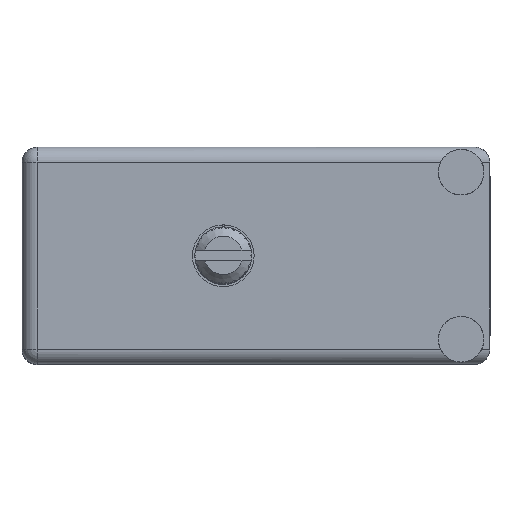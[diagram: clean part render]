
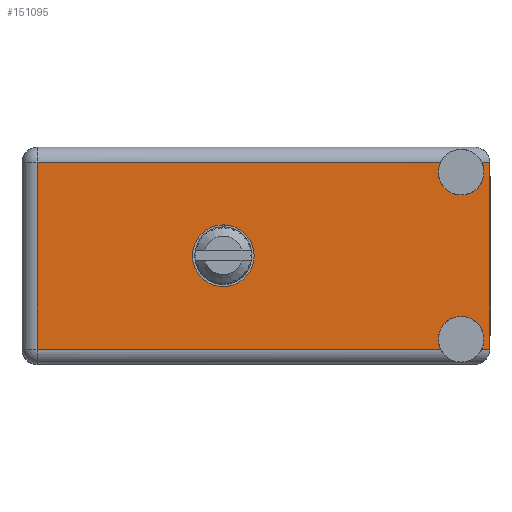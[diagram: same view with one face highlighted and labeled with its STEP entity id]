
A CAD part, top view. The second image highlights one B-rep face of the part: STEP entity #151095.
In plain terms, the highlighted face is planar.
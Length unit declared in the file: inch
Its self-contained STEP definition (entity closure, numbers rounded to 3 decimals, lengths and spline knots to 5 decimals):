
#596 = CARTESIAN_POINT ( 'NONE',  ( 1.37741, 0.906, -0.05 ) ) ;
#1557 = CARTESIAN_POINT ( 'NONE',  ( 0.6625, 0.906, -0.256 ) ) ;
#2909 = LINE ( 'NONE', #73271, #151049 ) ;
#3049 = DIRECTION ( 'NONE',  ( 0., 1., 0. ) ) ;
#3292 = CARTESIAN_POINT ( 'NONE',  ( 0.6625, 0.906, -0.3575 ) ) ;
#5131 = LINE ( 'NONE', #38568, #133045 ) ;
#6675 = ORIENTED_EDGE ( 'NONE', *, *, #41124, .T. ) ;
#7584 = VERTEX_POINT ( 'NONE', #131062 ) ;
#11109 = DIRECTION ( 'NONE',  ( 0., 1., 0. ) ) ;
#11494 = ORIENTED_EDGE ( 'NONE', *, *, #96098, .T. ) ;
#16154 = LINE ( 'NONE', #109413, #182245 ) ;
#17446 = DIRECTION ( 'NONE',  ( 0., 0., 1. ) ) ;
#20794 = DIRECTION ( 'NONE',  ( 0., 1., 0. ) ) ;
#22170 = ORIENTED_EDGE ( 'NONE', *, *, #29970, .T. ) ;
#28681 = ORIENTED_EDGE ( 'NONE', *, *, #48015, .F. ) ;
#28885 = VERTEX_POINT ( 'NONE', #99645 ) ;
#29970 = EDGE_CURVE ( 'NONE', #140337, #28885, #2909, .T. ) ;
#32142 = DIRECTION ( 'NONE',  ( 0., 1., 0. ) ) ;
#35835 = VERTEX_POINT ( 'NONE', #596 ) ;
#36624 = AXIS2_PLACEMENT_3D ( 'NONE', #179896, #63413, #94110 ) ;
#38568 = CARTESIAN_POINT ( 'NONE',  ( 0.05, 0.906, -0.715 ) ) ;
#41124 = EDGE_CURVE ( 'NONE', #153997, #7584, #5131, .T. ) ;
#47847 = CARTESIAN_POINT ( 'NONE',  ( 0.6625, 0.906, -0.3575 ) ) ;
#47983 = EDGE_CURVE ( 'NONE', #53860, #103838, #131945, .T. ) ;
#48015 = EDGE_CURVE ( 'NONE', #103838, #53860, #111901, .T. ) ;
#53860 = VERTEX_POINT ( 'NONE', #160306 ) ;
#54438 = CARTESIAN_POINT ( 'NONE',  ( 1.445, 0.906, -0.0825 ) ) ;
#57145 = AXIS2_PLACEMENT_3D ( 'NONE', #54438, #184155, #113377 ) ;
#57504 = EDGE_LOOP ( 'NONE', ( #11494, #119751, #124812, #22170, #175288, #134288, #147237, #143438, #183204, #6675 ) ) ;
#58439 = PLANE ( 'NONE',  #61198 ) ;
#58779 = VERTEX_POINT ( 'NONE', #172101 ) ;
#60140 = EDGE_CURVE ( 'NONE', #146361, #66813, #97274, .T. ) ;
#61198 = AXIS2_PLACEMENT_3D ( 'NONE', #173760, #32142, #174386 ) ;
#61536 = VECTOR ( 'NONE', #171628, 39.37008 ) ;
#62632 = CARTESIAN_POINT ( 'NONE',  ( 1.445, 0.906, -0.6325 ) ) ;
#62812 = AXIS2_PLACEMENT_3D ( 'NONE', #3292, #87406, #103688 ) ;
#63413 = DIRECTION ( 'NONE',  ( 0., 1., 0. ) ) ;
#66813 = VERTEX_POINT ( 'NONE', #106801 ) ;
#69987 = CARTESIAN_POINT ( 'NONE',  ( 1.539, 0.906, 0. ) ) ;
#70924 = CARTESIAN_POINT ( 'NONE',  ( 1.445, 0.906, -0.5575 ) ) ;
#73271 = CARTESIAN_POINT ( 'NONE',  ( 1.539, 0.906, -0.05 ) ) ;
#79541 = FACE_OUTER_BOUND ( 'NONE', #57504, .T. ) ;
#80085 = ORIENTED_EDGE ( 'NONE', *, *, #47983, .F. ) ;
#83356 = CARTESIAN_POINT ( 'NONE',  ( 1.539, 0.906, -0.05 ) ) ;
#87406 = DIRECTION ( 'NONE',  ( 0., 1., 0. ) ) ;
#87454 = EDGE_CURVE ( 'NONE', #120248, #28885, #135695, .T. ) ;
#91360 = CARTESIAN_POINT ( 'NONE',  ( 1.539, 0.906, -0.665 ) ) ;
#91677 = AXIS2_PLACEMENT_3D ( 'NONE', #47847, #20794, #121111 ) ;
#94110 = DIRECTION ( 'NONE',  ( 0., 0., 1. ) ) ;
#95223 = LINE ( 'NONE', #83356, #61536 ) ;
#96098 = EDGE_CURVE ( 'NONE', #7584, #35835, #95223, .T. ) ;
#97105 = CARTESIAN_POINT ( 'NONE',  ( 1.445, 0.906, -0.6325 ) ) ;
#97274 = CIRCLE ( 'NONE', #147694, 0.075 ) ;
#97648 = VECTOR ( 'NONE', #174543, 39.37008 ) ;
#99366 = EDGE_CURVE ( 'NONE', #140337, #152375, #117106, .T. ) ;
#99645 = CARTESIAN_POINT ( 'NONE',  ( 1.539, 0.906, -0.05 ) ) ;
#103688 = DIRECTION ( 'NONE',  ( 0., 0., 1. ) ) ;
#103838 = VERTEX_POINT ( 'NONE', #1557 ) ;
#106801 = CARTESIAN_POINT ( 'NONE',  ( 1.51259, 0.906, -0.665 ) ) ;
#108058 = LINE ( 'NONE', #149409, #177628 ) ;
#109413 = CARTESIAN_POINT ( 'NONE',  ( 0., 0.906, -0.665 ) ) ;
#111489 = DIRECTION ( 'NONE',  ( 0., 0., 1. ) ) ;
#111901 = CIRCLE ( 'NONE', #91677, 0.1015 ) ;
#113377 = DIRECTION ( 'NONE',  ( 0., 0., 1. ) ) ;
#117106 = CIRCLE ( 'NONE', #36624, 0.075 ) ;
#119751 = ORIENTED_EDGE ( 'NONE', *, *, #128968, .F. ) ;
#120248 = VERTEX_POINT ( 'NONE', #91360 ) ;
#121111 = DIRECTION ( 'NONE',  ( 0., 0., 1. ) ) ;
#124812 = ORIENTED_EDGE ( 'NONE', *, *, #99366, .F. ) ;
#128968 = EDGE_CURVE ( 'NONE', #152375, #35835, #153429, .T. ) ;
#131062 = CARTESIAN_POINT ( 'NONE',  ( 0.05, 0.906, -0.05 ) ) ;
#131945 = CIRCLE ( 'NONE', #62812, 0.1015 ) ;
#133045 = VECTOR ( 'NONE', #153852, 39.37008 ) ;
#133136 = CARTESIAN_POINT ( 'NONE',  ( 1.445, 0.906, -0.1575 ) ) ;
#134288 = ORIENTED_EDGE ( 'NONE', *, *, #142106, .T. ) ;
#135695 = LINE ( 'NONE', #69987, #97648 ) ;
#139358 = AXIS2_PLACEMENT_3D ( 'NONE', #62632, #3049, #17446 ) ;
#140337 = VERTEX_POINT ( 'NONE', #160698 ) ;
#142106 = EDGE_CURVE ( 'NONE', #120248, #66813, #16154, .T. ) ;
#143438 = ORIENTED_EDGE ( 'NONE', *, *, #182473, .F. ) ;
#146361 = VERTEX_POINT ( 'NONE', #70924 ) ;
#147237 = ORIENTED_EDGE ( 'NONE', *, *, #60140, .F. ) ;
#147694 = AXIS2_PLACEMENT_3D ( 'NONE', #97105, #11109, #111489 ) ;
#149409 = CARTESIAN_POINT ( 'NONE',  ( 0., 0.906, -0.665 ) ) ;
#151049 = VECTOR ( 'NONE', #162791, 39.37008 ) ;
#151095 = ADVANCED_FACE ( 'NONE', ( #168203, #79541 ), #58439, .T. ) ;
#152375 = VERTEX_POINT ( 'NONE', #133136 ) ;
#152613 = DIRECTION ( 'NONE',  ( -1., 0., 0. ) ) ;
#153429 = CIRCLE ( 'NONE', #57145, 0.075 ) ;
#153852 = DIRECTION ( 'NONE',  ( 0., 0., 1. ) ) ;
#153997 = VERTEX_POINT ( 'NONE', #170216 ) ;
#154601 = CIRCLE ( 'NONE', #139358, 0.075 ) ;
#160306 = CARTESIAN_POINT ( 'NONE',  ( 0.6625, 0.906, -0.459 ) ) ;
#160698 = CARTESIAN_POINT ( 'NONE',  ( 1.51259, 0.906, -0.05 ) ) ;
#162791 = DIRECTION ( 'NONE',  ( 1., 0., 0. ) ) ;
#168203 = FACE_BOUND ( 'NONE', #168515, .T. ) ;
#168515 = EDGE_LOOP ( 'NONE', ( #28681, #80085 ) ) ;
#170216 = CARTESIAN_POINT ( 'NONE',  ( 0.05, 0.906, -0.665 ) ) ;
#171628 = DIRECTION ( 'NONE',  ( 1., 0., 0. ) ) ;
#172101 = CARTESIAN_POINT ( 'NONE',  ( 1.37741, 0.906, -0.665 ) ) ;
#173760 = CARTESIAN_POINT ( 'NONE',  ( 0., 0.906, -0.715 ) ) ;
#174386 = DIRECTION ( 'NONE',  ( 0., 0., 1. ) ) ;
#174543 = DIRECTION ( 'NONE',  ( 0., 0., 1. ) ) ;
#175288 = ORIENTED_EDGE ( 'NONE', *, *, #87454, .F. ) ;
#177628 = VECTOR ( 'NONE', #180008, 39.37008 ) ;
#179795 = EDGE_CURVE ( 'NONE', #58779, #153997, #108058, .T. ) ;
#179896 = CARTESIAN_POINT ( 'NONE',  ( 1.445, 0.906, -0.0825 ) ) ;
#180008 = DIRECTION ( 'NONE',  ( -1., 0., 0. ) ) ;
#182245 = VECTOR ( 'NONE', #152613, 39.37008 ) ;
#182473 = EDGE_CURVE ( 'NONE', #58779, #146361, #154601, .T. ) ;
#183204 = ORIENTED_EDGE ( 'NONE', *, *, #179795, .T. ) ;
#184155 = DIRECTION ( 'NONE',  ( 0., 1., 0. ) ) ;
